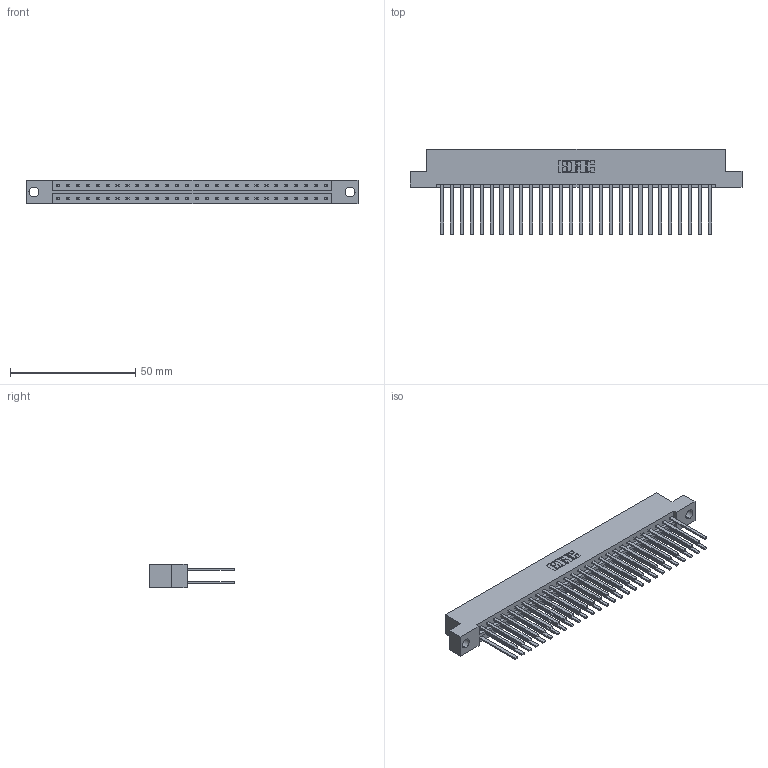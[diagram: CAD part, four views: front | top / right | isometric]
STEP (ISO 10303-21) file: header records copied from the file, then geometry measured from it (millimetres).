
FILE_DESCRIPTION (( 'STEP AP203' ), '1' );
FILE_NAME ('333-056-544-204.STEP', '2018-08-04T05:03:31', ( '' ), ( '' ), 'SwSTEP 2.0', 'SolidWorks 2016', '' );
FILE_SCHEMA (( 'CONFIG_CONTROL_DESIGN' ));
Length unit declared in the file: inch
Products named in the file (3): 345-292-001_345-293-144; 333-056-544-204; 333 Part_Flush - .156 Dia - TH
Assembly tree (57 placements, depth 2):
  333-056-544-204
    333 Part_Flush - .156 Dia - TH
    345-292-001_345-293-144  x56
Bounding box: 132.49 x 34.3 x 9.4 mm (x, y, z)
Volume: 14092.3 mm3; surface area: 18837.2 mm2
Topology: 57 solids, 57 shells, 2690 faces, 7983 edges, 5246 vertices
Faces by surface type: plane 1862, cylinder 828
Entity records: 19643 total; most frequent: CARTESIAN_POINT 3270, ORIENTED_EDGE 3206, DIRECTION 2815, EDGE_CURVE 1603, VECTOR 1479, LINE 1479, VERTEX_POINT 1066, AXIS2_PLACEMENT_3D 668
